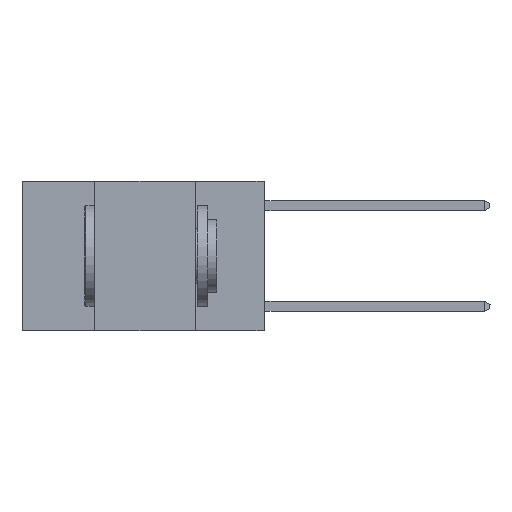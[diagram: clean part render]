
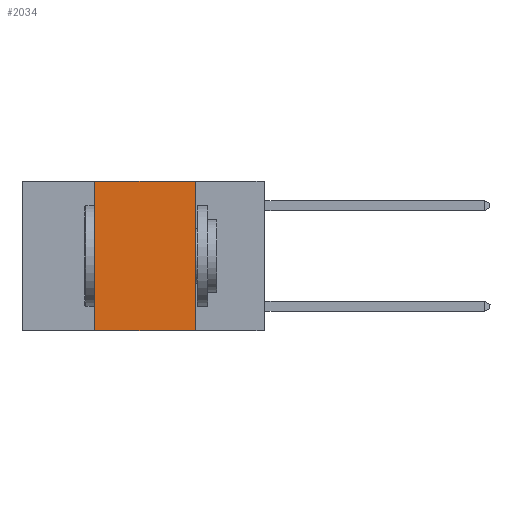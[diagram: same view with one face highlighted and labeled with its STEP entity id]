
A CAD part, left-side view. The second image highlights one B-rep face of the part: STEP entity #2034.
In plain terms, the highlighted planar face has unit normal (-1, 0, 0).
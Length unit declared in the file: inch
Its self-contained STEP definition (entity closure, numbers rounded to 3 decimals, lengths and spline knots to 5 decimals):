
#2034 = ADVANCED_FACE ( 'NONE', ( #3400 ), #8930, .F. ) ;
#3122 = ORIENTED_EDGE ( 'NONE', *, *, #22310, .F. ) ;
#3335 = LINE ( 'NONE', #15679, #8092 ) ;
#3400 = FACE_OUTER_BOUND ( 'NONE', #20531, .T. ) ;
#4188 = EDGE_CURVE ( 'NONE', #20197, #21331, #3335, .T. ) ;
#5601 = CARTESIAN_POINT ( 'NONE',  ( 0., 0.17, 0. ) ) ;
#5639 = DIRECTION ( 'NONE',  ( 0., 0., -1. ) ) ;
#5678 = VERTEX_POINT ( 'NONE', #21761 ) ;
#7339 = VECTOR ( 'NONE', #12201, 39.37008 ) ;
#7901 = CARTESIAN_POINT ( 'NONE',  ( 0., 0.42, 0. ) ) ;
#8092 = VECTOR ( 'NONE', #5639, 39.37008 ) ;
#8240 = CARTESIAN_POINT ( 'NONE',  ( 0., 0.6, 0. ) ) ;
#8520 = AXIS2_PLACEMENT_3D ( 'NONE', #20561, #20068, #20063 ) ;
#8930 = PLANE ( 'NONE',  #8520 ) ;
#9242 = CARTESIAN_POINT ( 'NONE',  ( 0., 0.17, -0.37 ) ) ;
#10157 = CARTESIAN_POINT ( 'NONE',  ( 0., 0.42, 0. ) ) ;
#10231 = LINE ( 'NONE', #8240, #15572 ) ;
#10264 = DIRECTION ( 'NONE',  ( 0., -1., 0. ) ) ;
#10291 = VECTOR ( 'NONE', #23797, 39.37008 ) ;
#11563 = EDGE_CURVE ( 'NONE', #21583, #20197, #10231, .T. ) ;
#11756 = CARTESIAN_POINT ( 'NONE',  ( 0., 0.6, -0.37 ) ) ;
#12073 = LINE ( 'NONE', #10157, #7339 ) ;
#12201 = DIRECTION ( 'NONE',  ( 0., 0., 1. ) ) ;
#14374 = ORIENTED_EDGE ( 'NONE', *, *, #11563, .F. ) ;
#15416 = ORIENTED_EDGE ( 'NONE', *, *, #18187, .T. ) ;
#15572 = VECTOR ( 'NONE', #10264, 39.37008 ) ;
#15679 = CARTESIAN_POINT ( 'NONE',  ( 0., 0.17, 0. ) ) ;
#18187 = EDGE_CURVE ( 'NONE', #5678, #21331, #20978, .T. ) ;
#20063 = DIRECTION ( 'NONE',  ( 0., 0., -1. ) ) ;
#20068 = DIRECTION ( 'NONE',  ( 1., 0., 0. ) ) ;
#20197 = VERTEX_POINT ( 'NONE', #5601 ) ;
#20531 = EDGE_LOOP ( 'NONE', ( #21657, #14374, #3122, #15416 ) ) ;
#20561 = CARTESIAN_POINT ( 'NONE',  ( 0., 0.6, 0. ) ) ;
#20978 = LINE ( 'NONE', #11756, #10291 ) ;
#21331 = VERTEX_POINT ( 'NONE', #9242 ) ;
#21583 = VERTEX_POINT ( 'NONE', #7901 ) ;
#21657 = ORIENTED_EDGE ( 'NONE', *, *, #4188, .F. ) ;
#21761 = CARTESIAN_POINT ( 'NONE',  ( 0., 0.42, -0.37 ) ) ;
#22310 = EDGE_CURVE ( 'NONE', #5678, #21583, #12073, .T. ) ;
#23797 = DIRECTION ( 'NONE',  ( 0., -1., 0. ) ) ;
